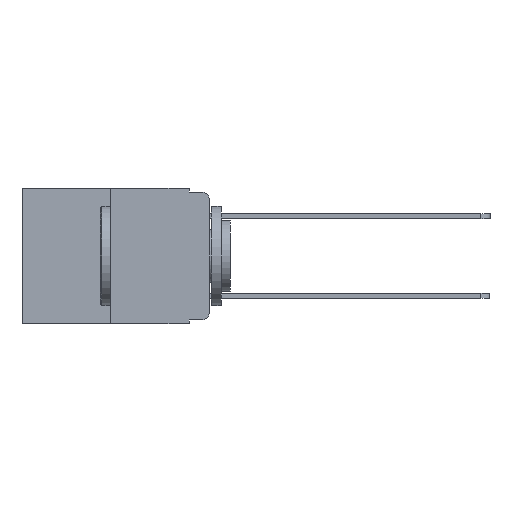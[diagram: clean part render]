
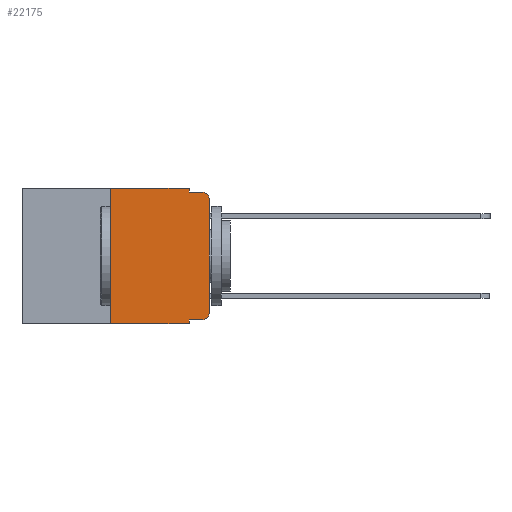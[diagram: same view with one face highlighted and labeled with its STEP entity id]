
A CAD part, left-side view. The second image highlights one B-rep face of the part: STEP entity #22175.
In plain terms, the highlighted planar face has unit normal (-1, 0, 0).
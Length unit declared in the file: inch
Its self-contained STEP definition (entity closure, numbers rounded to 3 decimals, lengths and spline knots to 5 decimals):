
#499 = VERTEX_POINT ( 'NONE', #7705 ) ;
#567 = VERTEX_POINT ( 'NONE', #18760 ) ;
#883 = FACE_OUTER_BOUND ( 'NONE', #17953, .T. ) ;
#1208 = DIRECTION ( 'NONE',  ( 0., -1., 0. ) ) ;
#1268 = LINE ( 'NONE', #1409, #21729 ) ;
#1272 = DIRECTION ( 'NONE',  ( 0., 0., -1. ) ) ;
#1373 = VECTOR ( 'NONE', #9782, 39.37008 ) ;
#1409 = CARTESIAN_POINT ( 'NONE',  ( 0., 0.051, 0. ) ) ;
#1499 = VERTEX_POINT ( 'NONE', #6280 ) ;
#2146 = VECTOR ( 'NONE', #13881, 39.37008 ) ;
#2334 = CARTESIAN_POINT ( 'NONE',  ( 0., 0.02, -0.313 ) ) ;
#2366 = ORIENTED_EDGE ( 'NONE', *, *, #25654, .F. ) ;
#2683 = ORIENTED_EDGE ( 'NONE', *, *, #19746, .F. ) ;
#2790 = LINE ( 'NONE', #11182, #16093 ) ;
#3107 = CARTESIAN_POINT ( 'NONE',  ( 0., 0.051, -0.01 ) ) ;
#3152 = PLANE ( 'NONE',  #17799 ) ;
#3177 = DIRECTION ( 'NONE',  ( 0., -1., 0. ) ) ;
#3469 = DIRECTION ( 'NONE',  ( 0., 0., -1. ) ) ;
#3983 = CARTESIAN_POINT ( 'NONE',  ( 0., 0., -0.03 ) ) ;
#4044 = VERTEX_POINT ( 'NONE', #23219 ) ;
#4110 = VECTOR ( 'NONE', #3177, 39.37008 ) ;
#4277 = ORIENTED_EDGE ( 'NONE', *, *, #15933, .T. ) ;
#4349 = DIRECTION ( 'NONE',  ( 0., 0., -1. ) ) ;
#4368 = CIRCLE ( 'NONE', #22387, 0.02 ) ;
#4610 = VERTEX_POINT ( 'NONE', #21038 ) ;
#4632 = DIRECTION ( 'NONE',  ( -1., 0., 0. ) ) ;
#4773 = VERTEX_POINT ( 'NONE', #3107 ) ;
#6280 = CARTESIAN_POINT ( 'NONE',  ( 0., 0.051, -0.333 ) ) ;
#6409 = ORIENTED_EDGE ( 'NONE', *, *, #21376, .F. ) ;
#6449 = DIRECTION ( 'NONE',  ( 0., 0., 1. ) ) ;
#6724 = ORIENTED_EDGE ( 'NONE', *, *, #15895, .T. ) ;
#6984 = EDGE_CURVE ( 'NONE', #19130, #7450, #4368, .T. ) ;
#7450 = VERTEX_POINT ( 'NONE', #16207 ) ;
#7705 = CARTESIAN_POINT ( 'NONE',  ( 0., 0.051, 0. ) ) ;
#7929 = CARTESIAN_POINT ( 'NONE',  ( 0., 0., 0. ) ) ;
#8479 = VERTEX_POINT ( 'NONE', #16792 ) ;
#8620 = EDGE_CURVE ( 'NONE', #499, #4773, #1268, .T. ) ;
#8746 = LINE ( 'NONE', #15044, #4110 ) ;
#9782 = DIRECTION ( 'NONE',  ( 0., 0., -1. ) ) ;
#10143 = ORIENTED_EDGE ( 'NONE', *, *, #19780, .T. ) ;
#10832 = LINE ( 'NONE', #21878, #15478 ) ;
#11182 = CARTESIAN_POINT ( 'NONE',  ( 0., 0.051, -0.333 ) ) ;
#11659 = CARTESIAN_POINT ( 'NONE',  ( 0., 0.051, 0. ) ) ;
#11977 = ORIENTED_EDGE ( 'NONE', *, *, #6984, .T. ) ;
#12080 = LINE ( 'NONE', #7929, #2146 ) ;
#12088 = EDGE_CURVE ( 'NONE', #8479, #499, #12919, .T. ) ;
#12574 = LINE ( 'NONE', #11659, #1373 ) ;
#12919 = LINE ( 'NONE', #17112, #17557 ) ;
#13198 = DIRECTION ( 'NONE',  ( 1., 0., 0. ) ) ;
#13714 = LINE ( 'NONE', #16318, #18342 ) ;
#13881 = DIRECTION ( 'NONE',  ( 0., 0., 1. ) ) ;
#14862 = CIRCLE ( 'NONE', #22796, 0.02 ) ;
#15044 = CARTESIAN_POINT ( 'NONE',  ( 0., 0.473, -0.343 ) ) ;
#15478 = VECTOR ( 'NONE', #23854, 39.37008 ) ;
#15895 = EDGE_CURVE ( 'NONE', #567, #19130, #12080, .T. ) ;
#15933 = EDGE_CURVE ( 'NONE', #1499, #4610, #2790, .T. ) ;
#15944 = DIRECTION ( 'NONE',  ( 0., -1., 0. ) ) ;
#16093 = VECTOR ( 'NONE', #15944, 39.37008 ) ;
#16189 = DIRECTION ( 'NONE',  ( -1., 0., 0. ) ) ;
#16207 = CARTESIAN_POINT ( 'NONE',  ( 0., 0.02, -0.01 ) ) ;
#16318 = CARTESIAN_POINT ( 'NONE',  ( 0., 0.25, 0. ) ) ;
#16483 = CARTESIAN_POINT ( 'NONE',  ( 0., 0.02, -0.03 ) ) ;
#16792 = CARTESIAN_POINT ( 'NONE',  ( 0., 0.25, 0. ) ) ;
#16957 = ORIENTED_EDGE ( 'NONE', *, *, #21607, .T. ) ;
#17078 = CARTESIAN_POINT ( 'NONE',  ( 0., 0.473, 0. ) ) ;
#17112 = CARTESIAN_POINT ( 'NONE',  ( 0., 0.473, 0. ) ) ;
#17557 = VECTOR ( 'NONE', #1208, 39.37008 ) ;
#17799 = AXIS2_PLACEMENT_3D ( 'NONE', #17078, #13198, #1272 ) ;
#17953 = EDGE_LOOP ( 'NONE', ( #6724, #11977, #2683, #24323, #20959, #6409, #16957, #2366, #4277, #10143 ) ) ;
#18342 = VECTOR ( 'NONE', #6449, 39.37008 ) ;
#18483 = DIRECTION ( 'NONE',  ( 0., 0., -1. ) ) ;
#18760 = CARTESIAN_POINT ( 'NONE',  ( 0., 0., -0.313 ) ) ;
#19130 = VERTEX_POINT ( 'NONE', #3983 ) ;
#19746 = EDGE_CURVE ( 'NONE', #4773, #7450, #10832, .T. ) ;
#19780 = EDGE_CURVE ( 'NONE', #4610, #567, #14862, .T. ) ;
#20959 = ORIENTED_EDGE ( 'NONE', *, *, #12088, .F. ) ;
#21038 = CARTESIAN_POINT ( 'NONE',  ( 0., 0.02, -0.333 ) ) ;
#21376 = EDGE_CURVE ( 'NONE', #24872, #8479, #13714, .T. ) ;
#21607 = EDGE_CURVE ( 'NONE', #24872, #4044, #8746, .T. ) ;
#21729 = VECTOR ( 'NONE', #3469, 39.37008 ) ;
#21878 = CARTESIAN_POINT ( 'NONE',  ( 0., 0.051, -0.01 ) ) ;
#21883 = CARTESIAN_POINT ( 'NONE',  ( 0., 0.25, -0.343 ) ) ;
#22175 = ADVANCED_FACE ( 'NONE', ( #883 ), #3152, .F. ) ;
#22387 = AXIS2_PLACEMENT_3D ( 'NONE', #16483, #4632, #18483 ) ;
#22796 = AXIS2_PLACEMENT_3D ( 'NONE', #2334, #16189, #4349 ) ;
#23219 = CARTESIAN_POINT ( 'NONE',  ( 0., 0.051, -0.343 ) ) ;
#23854 = DIRECTION ( 'NONE',  ( 0., -1., 0. ) ) ;
#24323 = ORIENTED_EDGE ( 'NONE', *, *, #8620, .F. ) ;
#24872 = VERTEX_POINT ( 'NONE', #21883 ) ;
#25654 = EDGE_CURVE ( 'NONE', #1499, #4044, #12574, .T. ) ;
